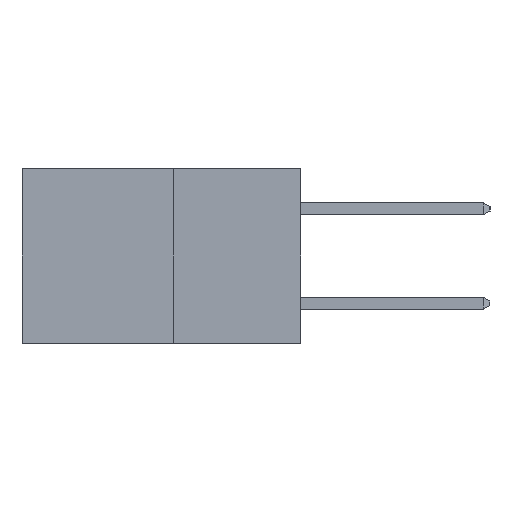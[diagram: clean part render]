
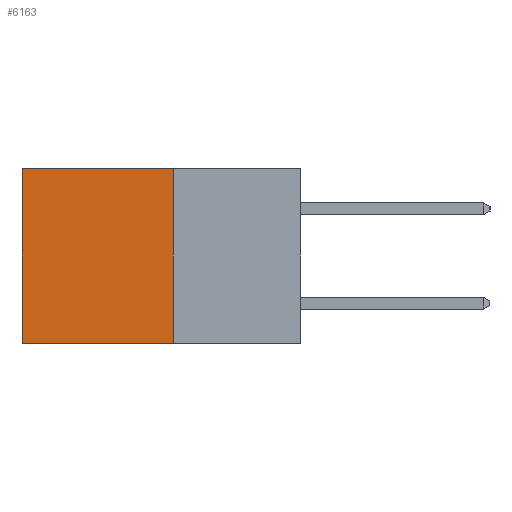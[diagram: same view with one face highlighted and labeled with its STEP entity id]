
A CAD part, left-side view. The second image highlights one B-rep face of the part: STEP entity #6163.
In plain terms, the highlighted planar face has unit normal (-1, 0, 0).
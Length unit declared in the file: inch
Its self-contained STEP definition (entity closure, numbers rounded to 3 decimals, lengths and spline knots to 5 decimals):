
#324 = VERTEX_POINT ( 'NONE', #3034 ) ;
#782 = VECTOR ( 'NONE', #5654, 39.37008 ) ;
#908 = DIRECTION ( 'NONE',  ( 0., 0., -1. ) ) ;
#910 = DIRECTION ( 'NONE',  ( 1., 0., 0. ) ) ;
#920 = CARTESIAN_POINT ( 'NONE',  ( 0.277, 0.27, -0.37 ) ) ;
#929 = PLANE ( 'NONE',  #4081 ) ;
#1168 = VECTOR ( 'NONE', #7328, 39.37008 ) ;
#2956 = LINE ( 'NONE', #6455, #782 ) ;
#3034 = CARTESIAN_POINT ( 'NONE',  ( 0.277, 0.59, -0.37 ) ) ;
#3178 = ORIENTED_EDGE ( 'NONE', *, *, #4084, .T. ) ;
#3683 = FACE_OUTER_BOUND ( 'NONE', #9512, .T. ) ;
#4081 = AXIS2_PLACEMENT_3D ( 'NONE', #920, #910, #908 ) ;
#4084 = EDGE_CURVE ( 'NONE', #9504, #7381, #2956, .T. ) ;
#4284 = EDGE_CURVE ( 'NONE', #9504, #4361, #7261, .T. ) ;
#4361 = VERTEX_POINT ( 'NONE', #5747 ) ;
#4719 = VECTOR ( 'NONE', #9356, 39.37008 ) ;
#4725 = EDGE_CURVE ( 'NONE', #4361, #324, #8705, .T. ) ;
#4868 = EDGE_CURVE ( 'NONE', #7381, #324, #9686, .T. ) ;
#4975 = CARTESIAN_POINT ( 'NONE',  ( 0.277, 0.27, 0. ) ) ;
#5065 = ORIENTED_EDGE ( 'NONE', *, *, #4725, .F. ) ;
#5320 = VECTOR ( 'NONE', #8243, 39.37008 ) ;
#5654 = DIRECTION ( 'NONE',  ( 0., 1., 0. ) ) ;
#5747 = CARTESIAN_POINT ( 'NONE',  ( 0.277, 0.27, -0.37 ) ) ;
#6163 = ADVANCED_FACE ( 'NONE', ( #3683 ), #929, .F. ) ;
#6455 = CARTESIAN_POINT ( 'NONE',  ( 0.277, 0.27, 0. ) ) ;
#6889 = ORIENTED_EDGE ( 'NONE', *, *, #4868, .T. ) ;
#7118 = ORIENTED_EDGE ( 'NONE', *, *, #4284, .F. ) ;
#7261 = LINE ( 'NONE', #7481, #1168 ) ;
#7328 = DIRECTION ( 'NONE',  ( 0., 0., -1. ) ) ;
#7381 = VERTEX_POINT ( 'NONE', #9832 ) ;
#7481 = CARTESIAN_POINT ( 'NONE',  ( 0.277, 0.27, -0.37 ) ) ;
#8221 = CARTESIAN_POINT ( 'NONE',  ( 0.277, 0.59, -0.37 ) ) ;
#8243 = DIRECTION ( 'NONE',  ( 0., 0., -1. ) ) ;
#8705 = LINE ( 'NONE', #9368, #4719 ) ;
#9356 = DIRECTION ( 'NONE',  ( 0., 1., 0. ) ) ;
#9368 = CARTESIAN_POINT ( 'NONE',  ( 0.277, 0.27, -0.37 ) ) ;
#9504 = VERTEX_POINT ( 'NONE', #4975 ) ;
#9512 = EDGE_LOOP ( 'NONE', ( #6889, #5065, #7118, #3178 ) ) ;
#9686 = LINE ( 'NONE', #8221, #5320 ) ;
#9832 = CARTESIAN_POINT ( 'NONE',  ( 0.277, 0.59, 0. ) ) ;
